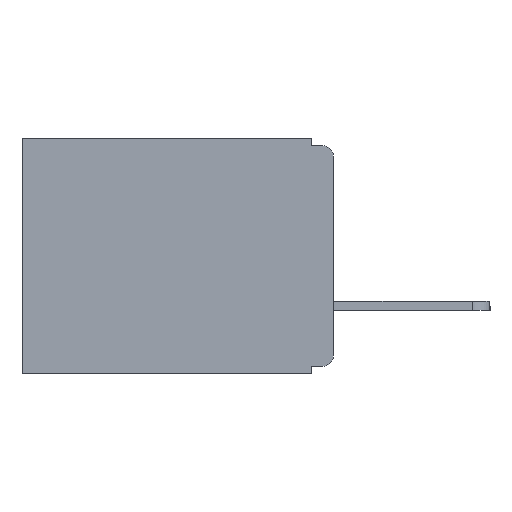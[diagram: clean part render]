
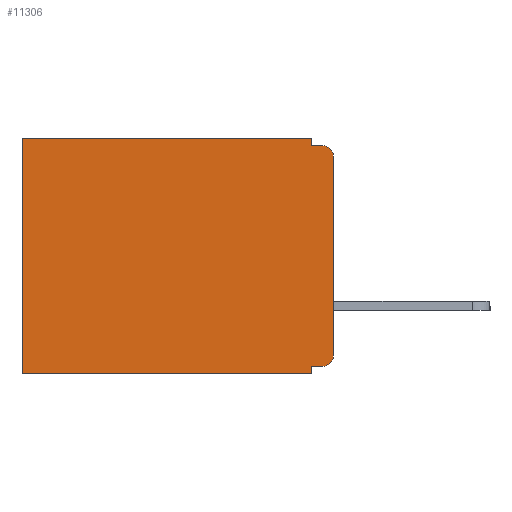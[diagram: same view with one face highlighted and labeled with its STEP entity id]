
A CAD part, left-side view. The second image highlights one B-rep face of the part: STEP entity #11306.
In plain terms, the highlighted planar face has unit normal (-1, 0, 0).
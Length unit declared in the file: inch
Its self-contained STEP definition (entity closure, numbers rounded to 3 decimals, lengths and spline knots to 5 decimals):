
#151 = VERTEX_POINT ( 'NONE', #24918 ) ;
#603 = EDGE_CURVE ( 'NONE', #15861, #25441, #28416, .T. ) ;
#1312 = VERTEX_POINT ( 'NONE', #9419 ) ;
#1518 = EDGE_CURVE ( 'NONE', #15839, #151, #17385, .T. ) ;
#1685 = CARTESIAN_POINT ( 'NONE',  ( 0.3, 0.031, 0. ) ) ;
#1994 = CARTESIAN_POINT ( 'NONE',  ( 0.3, 0., -0.33 ) ) ;
#2622 = DIRECTION ( 'NONE',  ( 0., 0., -1. ) ) ;
#2677 = ORIENTED_EDGE ( 'NONE', *, *, #18274, .F. ) ;
#3144 = EDGE_CURVE ( 'NONE', #27909, #1312, #29080, .T. ) ;
#3745 = ORIENTED_EDGE ( 'NONE', *, *, #18824, .T. ) ;
#4175 = CARTESIAN_POINT ( 'NONE',  ( 0.3, 0., -0.33 ) ) ;
#4983 = CARTESIAN_POINT ( 'NONE',  ( 0.3, 0., -0.33 ) ) ;
#5062 = LINE ( 'NONE', #4983, #10391 ) ;
#5165 = CARTESIAN_POINT ( 'NONE',  ( 0.3, 0.031, -0.32 ) ) ;
#5431 = AXIS2_PLACEMENT_3D ( 'NONE', #9811, #25692, #12117 ) ;
#5496 = CARTESIAN_POINT ( 'NONE',  ( 0.3, 0.015, -0.32 ) ) ;
#6142 = CARTESIAN_POINT ( 'NONE',  ( 0.3, 0., -0.025 ) ) ;
#6349 = VERTEX_POINT ( 'NONE', #8757 ) ;
#6546 = DIRECTION ( 'NONE',  ( 0., 0., -1. ) ) ;
#6566 = CARTESIAN_POINT ( 'NONE',  ( 0.3, 0.031, 0. ) ) ;
#7695 = DIRECTION ( 'NONE',  ( 0., 1., 0. ) ) ;
#7765 = LINE ( 'NONE', #12264, #19104 ) ;
#8757 = CARTESIAN_POINT ( 'NONE',  ( 0.3, 0.031, -0.01 ) ) ;
#9151 = AXIS2_PLACEMENT_3D ( 'NONE', #16297, #18926, #19371 ) ;
#9419 = CARTESIAN_POINT ( 'NONE',  ( 0.3, 0.031, -0.33 ) ) ;
#9811 = CARTESIAN_POINT ( 'NONE',  ( 0.3, 0.015, -0.305 ) ) ;
#9914 = VECTOR ( 'NONE', #20138, 39.37008 ) ;
#10274 = ORIENTED_EDGE ( 'NONE', *, *, #22895, .F. ) ;
#10391 = VECTOR ( 'NONE', #11762, 39.37008 ) ;
#10584 = ORIENTED_EDGE ( 'NONE', *, *, #1518, .T. ) ;
#11112 = VECTOR ( 'NONE', #2622, 39.37008 ) ;
#11306 = ADVANCED_FACE ( 'NONE', ( #20397 ), #17881, .F. ) ;
#11754 = VECTOR ( 'NONE', #27029, 39.37008 ) ;
#11762 = DIRECTION ( 'NONE',  ( 0., 0., -1. ) ) ;
#11840 = VERTEX_POINT ( 'NONE', #22474 ) ;
#12117 = DIRECTION ( 'NONE',  ( 0., 0., -1. ) ) ;
#12264 = CARTESIAN_POINT ( 'NONE',  ( 0.3, 0., -0.01 ) ) ;
#12686 = DIRECTION ( 'NONE',  ( 0., 1., 0. ) ) ;
#14193 = EDGE_CURVE ( 'NONE', #1312, #11840, #21280, .T. ) ;
#14553 = DIRECTION ( 'NONE',  ( 0., -1., 0. ) ) ;
#15839 = VERTEX_POINT ( 'NONE', #6142 ) ;
#15861 = VERTEX_POINT ( 'NONE', #1685 ) ;
#15937 = VERTEX_POINT ( 'NONE', #20135 ) ;
#16156 = VECTOR ( 'NONE', #7695, 39.37008 ) ;
#16297 = CARTESIAN_POINT ( 'NONE',  ( 0.3, 0.015, -0.025 ) ) ;
#17011 = ORIENTED_EDGE ( 'NONE', *, *, #14193, .F. ) ;
#17151 = LINE ( 'NONE', #18507, #11112 ) ;
#17385 = CIRCLE ( 'NONE', #9151, 0.015 ) ;
#17881 = PLANE ( 'NONE',  #20295 ) ;
#17902 = DIRECTION ( 'NONE',  ( 0., 0., -1. ) ) ;
#17906 = CIRCLE ( 'NONE', #5431, 0.015 ) ;
#18274 = EDGE_CURVE ( 'NONE', #25700, #27909, #26749, .T. ) ;
#18339 = CARTESIAN_POINT ( 'NONE',  ( 0.3, 0.437, 0. ) ) ;
#18449 = ORIENTED_EDGE ( 'NONE', *, *, #19966, .F. ) ;
#18507 = CARTESIAN_POINT ( 'NONE',  ( 0.3, 0.437, -0.33 ) ) ;
#18824 = EDGE_CURVE ( 'NONE', #25700, #15937, #17906, .T. ) ;
#18926 = DIRECTION ( 'NONE',  ( -1., 0., 0. ) ) ;
#19104 = VECTOR ( 'NONE', #14553, 39.37008 ) ;
#19371 = DIRECTION ( 'NONE',  ( 0., 0., -1. ) ) ;
#19822 = ORIENTED_EDGE ( 'NONE', *, *, #19931, .T. ) ;
#19931 = EDGE_CURVE ( 'NONE', #25441, #11840, #17151, .T. ) ;
#19966 = EDGE_CURVE ( 'NONE', #15839, #15937, #5062, .T. ) ;
#20133 = DIRECTION ( 'NONE',  ( 1., 0., 0. ) ) ;
#20135 = CARTESIAN_POINT ( 'NONE',  ( 0.3, 0., -0.305 ) ) ;
#20138 = DIRECTION ( 'NONE',  ( 0., 1., 0. ) ) ;
#20295 = AXIS2_PLACEMENT_3D ( 'NONE', #4175, #20133, #6546 ) ;
#20397 = FACE_OUTER_BOUND ( 'NONE', #22716, .T. ) ;
#20906 = ORIENTED_EDGE ( 'NONE', *, *, #3144, .F. ) ;
#21263 = CARTESIAN_POINT ( 'NONE',  ( 0.3, 0., -0.32 ) ) ;
#21280 = LINE ( 'NONE', #1994, #9914 ) ;
#21861 = VECTOR ( 'NONE', #17902, 39.37008 ) ;
#22396 = VECTOR ( 'NONE', #12686, 39.37008 ) ;
#22474 = CARTESIAN_POINT ( 'NONE',  ( 0.3, 0.437, -0.33 ) ) ;
#22716 = EDGE_LOOP ( 'NONE', ( #18449, #10584, #23772, #10274, #23412, #19822, #17011, #20906, #2677, #3745 ) ) ;
#22895 = EDGE_CURVE ( 'NONE', #15861, #6349, #29279, .T. ) ;
#23412 = ORIENTED_EDGE ( 'NONE', *, *, #603, .T. ) ;
#23772 = ORIENTED_EDGE ( 'NONE', *, *, #29228, .F. ) ;
#24918 = CARTESIAN_POINT ( 'NONE',  ( 0.3, 0.015, -0.01 ) ) ;
#25437 = CARTESIAN_POINT ( 'NONE',  ( 0.3, 0., 0. ) ) ;
#25441 = VERTEX_POINT ( 'NONE', #18339 ) ;
#25692 = DIRECTION ( 'NONE',  ( -1., 0., 0. ) ) ;
#25700 = VERTEX_POINT ( 'NONE', #5496 ) ;
#26749 = LINE ( 'NONE', #21263, #16156 ) ;
#26902 = CARTESIAN_POINT ( 'NONE',  ( 0.3, 0.031, -0.33 ) ) ;
#27029 = DIRECTION ( 'NONE',  ( 0., 0., -1. ) ) ;
#27909 = VERTEX_POINT ( 'NONE', #5165 ) ;
#28416 = LINE ( 'NONE', #25437, #22396 ) ;
#29080 = LINE ( 'NONE', #26902, #11754 ) ;
#29228 = EDGE_CURVE ( 'NONE', #6349, #151, #7765, .T. ) ;
#29279 = LINE ( 'NONE', #6566, #21861 ) ;
